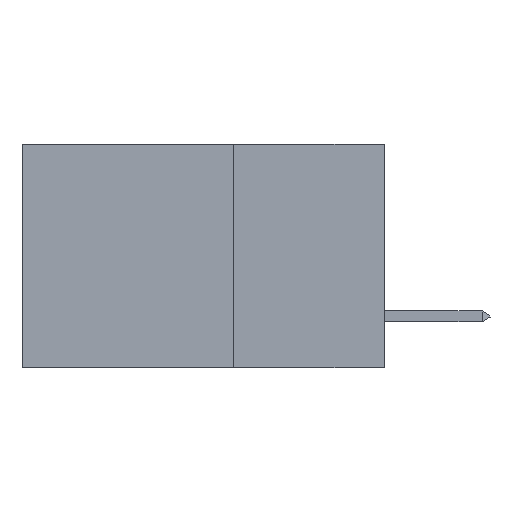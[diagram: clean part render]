
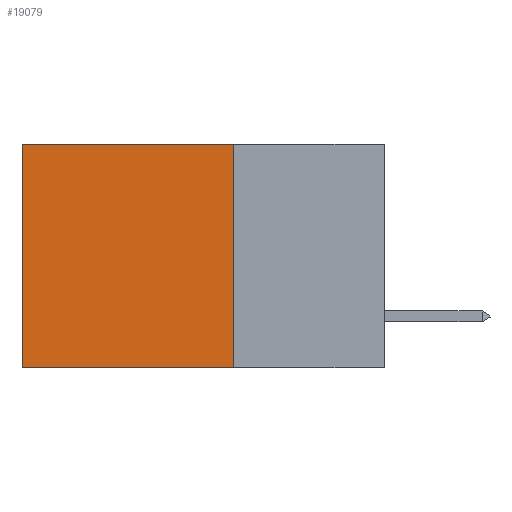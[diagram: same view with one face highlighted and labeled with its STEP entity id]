
A CAD part, left-side view. The second image highlights one B-rep face of the part: STEP entity #19079.
In plain terms, the highlighted planar face has unit normal (-1, 0, 0).
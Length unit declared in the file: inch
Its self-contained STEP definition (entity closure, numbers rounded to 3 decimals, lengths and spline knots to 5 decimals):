
#2517 = ORIENTED_EDGE ( 'NONE', *, *, #29304, .F. ) ;
#3578 = VECTOR ( 'NONE', #9571, 39.37008 ) ;
#4139 = DIRECTION ( 'NONE',  ( 0., 1., 0. ) ) ;
#4594 = ORIENTED_EDGE ( 'NONE', *, *, #14494, .T. ) ;
#6100 = VECTOR ( 'NONE', #31834, 39.37008 ) ;
#7117 = VECTOR ( 'NONE', #19197, 39.37008 ) ;
#9417 = ORIENTED_EDGE ( 'NONE', *, *, #27169, .F. ) ;
#9571 = DIRECTION ( 'NONE',  ( 0., 1., 0. ) ) ;
#9763 = CARTESIAN_POINT ( 'NONE',  ( 0.2875, 0.25, -0.37 ) ) ;
#11238 = PLANE ( 'NONE',  #15629 ) ;
#14494 = EDGE_CURVE ( 'NONE', #22220, #24082, #27832, .T. ) ;
#15423 = EDGE_LOOP ( 'NONE', ( #30200, #9417, #2517, #4594 ) ) ;
#15441 = CARTESIAN_POINT ( 'NONE',  ( 0.2875, 0.25, 0. ) ) ;
#15629 = AXIS2_PLACEMENT_3D ( 'NONE', #25426, #19811, #37167 ) ;
#17457 = EDGE_CURVE ( 'NONE', #24082, #29303, #36376, .T. ) ;
#18844 = FACE_OUTER_BOUND ( 'NONE', #15423, .T. ) ;
#18972 = CARTESIAN_POINT ( 'NONE',  ( 0.2875, 0.25, 0. ) ) ;
#19079 = ADVANCED_FACE ( 'NONE', ( #18844 ), #11238, .F. ) ;
#19197 = DIRECTION ( 'NONE',  ( 0., 0., -1. ) ) ;
#19404 = CARTESIAN_POINT ( 'NONE',  ( 0.2875, 0.6, 0. ) ) ;
#19811 = DIRECTION ( 'NONE',  ( 1., 0., 0. ) ) ;
#20225 = CARTESIAN_POINT ( 'NONE',  ( 0.2875, 0.6, -0.37 ) ) ;
#22220 = VERTEX_POINT ( 'NONE', #18972 ) ;
#23235 = CARTESIAN_POINT ( 'NONE',  ( 0.2875, 0.25, -0.37 ) ) ;
#24082 = VERTEX_POINT ( 'NONE', #19404 ) ;
#25426 = CARTESIAN_POINT ( 'NONE',  ( 0.2875, 0.25, 0. ) ) ;
#26231 = CARTESIAN_POINT ( 'NONE',  ( 0.2875, 0.25, 0. ) ) ;
#27169 = EDGE_CURVE ( 'NONE', #31570, #29303, #28843, .T. ) ;
#27764 = CARTESIAN_POINT ( 'NONE',  ( 0.2875, 0.6, 0. ) ) ;
#27832 = LINE ( 'NONE', #15441, #3578 ) ;
#28843 = LINE ( 'NONE', #9763, #35238 ) ;
#29303 = VERTEX_POINT ( 'NONE', #20225 ) ;
#29304 = EDGE_CURVE ( 'NONE', #22220, #31570, #37227, .T. ) ;
#30200 = ORIENTED_EDGE ( 'NONE', *, *, #17457, .T. ) ;
#31570 = VERTEX_POINT ( 'NONE', #23235 ) ;
#31834 = DIRECTION ( 'NONE',  ( 0., 0., -1. ) ) ;
#35238 = VECTOR ( 'NONE', #4139, 39.37008 ) ;
#36376 = LINE ( 'NONE', #27764, #7117 ) ;
#37167 = DIRECTION ( 'NONE',  ( 0., 0., -1. ) ) ;
#37227 = LINE ( 'NONE', #26231, #6100 ) ;
